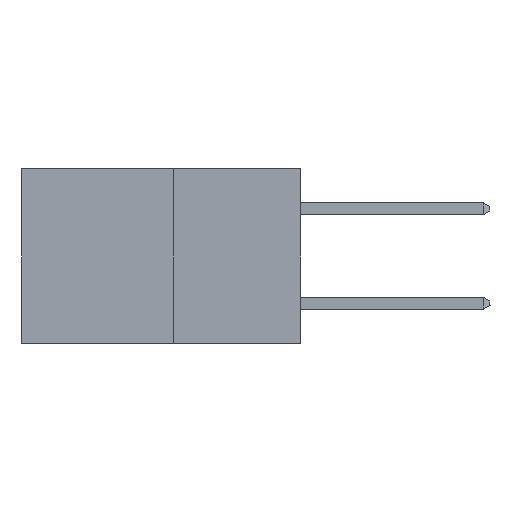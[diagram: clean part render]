
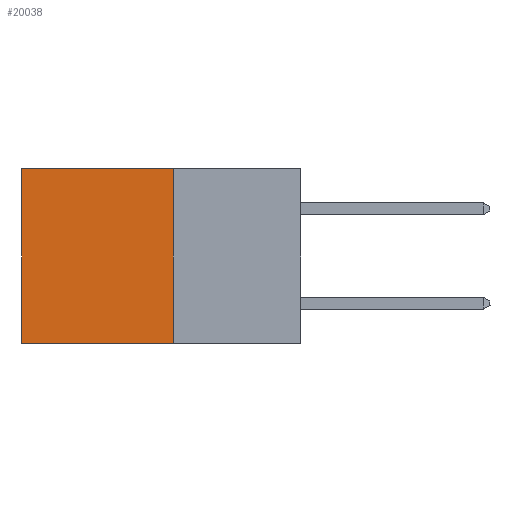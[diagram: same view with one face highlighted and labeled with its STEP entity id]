
A CAD part, left-side view. The second image highlights one B-rep face of the part: STEP entity #20038.
In plain terms, the highlighted planar face has unit normal (-1, 0, 0).
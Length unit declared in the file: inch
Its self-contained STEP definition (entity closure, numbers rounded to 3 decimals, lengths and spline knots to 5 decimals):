
#2602 = DIRECTION ( 'NONE',  ( 0., 1., 0. ) ) ;
#3171 = ORIENTED_EDGE ( 'NONE', *, *, #4390, .F. ) ;
#3234 = LINE ( 'NONE', #10445, #16732 ) ;
#3949 = LINE ( 'NONE', #17286, #17425 ) ;
#4390 = EDGE_CURVE ( 'NONE', #26258, #16299, #3234, .T. ) ;
#5195 = EDGE_CURVE ( 'NONE', #16299, #26330, #34283, .T. ) ;
#6937 = DIRECTION ( 'NONE',  ( 0., 0., -1. ) ) ;
#10445 = CARTESIAN_POINT ( 'NONE',  ( 0.277, 0.27, -0.37 ) ) ;
#11374 = CARTESIAN_POINT ( 'NONE',  ( 0.277, 0.59, 0. ) ) ;
#11924 = CARTESIAN_POINT ( 'NONE',  ( 0.277, 0.59, -0.37 ) ) ;
#12177 = CARTESIAN_POINT ( 'NONE',  ( 0.277, 0.27, -0.37 ) ) ;
#12915 = EDGE_CURVE ( 'NONE', #26258, #31248, #3949, .T. ) ;
#13116 = DIRECTION ( 'NONE',  ( 0., 0., -1. ) ) ;
#15349 = ORIENTED_EDGE ( 'NONE', *, *, #5195, .F. ) ;
#16299 = VERTEX_POINT ( 'NONE', #18341 ) ;
#16732 = VECTOR ( 'NONE', #13116, 39.37008 ) ;
#17286 = CARTESIAN_POINT ( 'NONE',  ( 0.277, 0.27, 0. ) ) ;
#17425 = VECTOR ( 'NONE', #27920, 39.37008 ) ;
#18341 = CARTESIAN_POINT ( 'NONE',  ( 0.277, 0.27, -0.37 ) ) ;
#18352 = LINE ( 'NONE', #29092, #25477 ) ;
#18843 = CARTESIAN_POINT ( 'NONE',  ( 0.277, 0.27, -0.37 ) ) ;
#19591 = CARTESIAN_POINT ( 'NONE',  ( 0.277, 0.27, 0. ) ) ;
#20038 = ADVANCED_FACE ( 'NONE', ( #32619 ), #20317, .F. ) ;
#20056 = VECTOR ( 'NONE', #2602, 39.37008 ) ;
#20317 = PLANE ( 'NONE',  #25009 ) ;
#23015 = DIRECTION ( 'NONE',  ( 1., 0., 0. ) ) ;
#24207 = ORIENTED_EDGE ( 'NONE', *, *, #30007, .T. ) ;
#25009 = AXIS2_PLACEMENT_3D ( 'NONE', #12177, #23015, #6937 ) ;
#25477 = VECTOR ( 'NONE', #31668, 39.37008 ) ;
#26258 = VERTEX_POINT ( 'NONE', #19591 ) ;
#26330 = VERTEX_POINT ( 'NONE', #11924 ) ;
#27920 = DIRECTION ( 'NONE',  ( 0., 1., 0. ) ) ;
#28762 = EDGE_LOOP ( 'NONE', ( #24207, #15349, #3171, #31468 ) ) ;
#29092 = CARTESIAN_POINT ( 'NONE',  ( 0.277, 0.59, -0.37 ) ) ;
#30007 = EDGE_CURVE ( 'NONE', #31248, #26330, #18352, .T. ) ;
#31248 = VERTEX_POINT ( 'NONE', #11374 ) ;
#31468 = ORIENTED_EDGE ( 'NONE', *, *, #12915, .T. ) ;
#31668 = DIRECTION ( 'NONE',  ( 0., 0., -1. ) ) ;
#32619 = FACE_OUTER_BOUND ( 'NONE', #28762, .T. ) ;
#34283 = LINE ( 'NONE', #18843, #20056 ) ;
